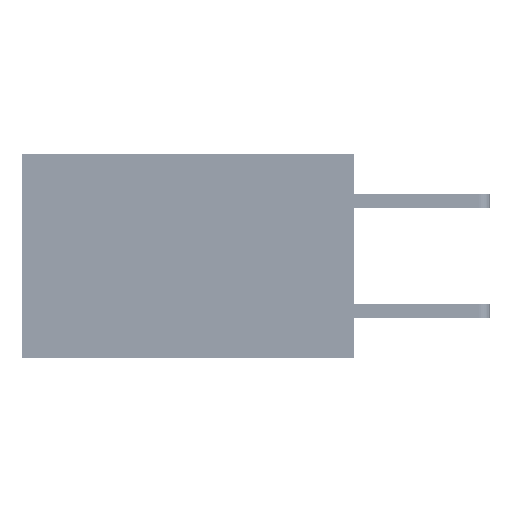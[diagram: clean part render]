
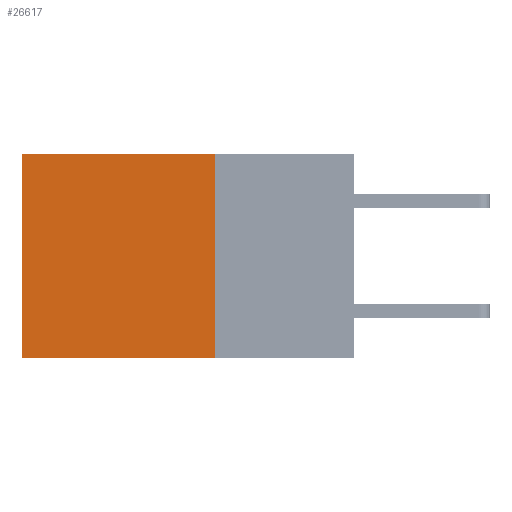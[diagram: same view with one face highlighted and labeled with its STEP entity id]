
A CAD part, left-side view. The second image highlights one B-rep face of the part: STEP entity #26617.
In plain terms, the highlighted planar face has unit normal (-1, 0, 0).
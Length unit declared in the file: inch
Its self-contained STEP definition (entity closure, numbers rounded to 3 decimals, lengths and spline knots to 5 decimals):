
#2583 = LINE ( 'NONE', #47488, #50290 ) ;
#2669 = CARTESIAN_POINT ( 'NONE',  ( 0.2875, 0.6, -0.37 ) ) ;
#3709 = EDGE_CURVE ( 'NONE', #24213, #41775, #29085, .T. ) ;
#3801 = CARTESIAN_POINT ( 'NONE',  ( 0.2875, 0.25, -0.37 ) ) ;
#5048 = DIRECTION ( 'NONE',  ( 0., 1., 0. ) ) ;
#6893 = ORIENTED_EDGE ( 'NONE', *, *, #13552, .F. ) ;
#9048 = LINE ( 'NONE', #33098, #9202 ) ;
#9202 = VECTOR ( 'NONE', #20428, 39.37008 ) ;
#13143 = ORIENTED_EDGE ( 'NONE', *, *, #35136, .T. ) ;
#13552 = EDGE_CURVE ( 'NONE', #24550, #24213, #2583, .T. ) ;
#14744 = VECTOR ( 'NONE', #5048, 39.37008 ) ;
#20428 = DIRECTION ( 'NONE',  ( 0., 0., -1. ) ) ;
#23697 = EDGE_CURVE ( 'NONE', #24550, #23934, #39280, .T. ) ;
#23934 = VERTEX_POINT ( 'NONE', #37385 ) ;
#24213 = VERTEX_POINT ( 'NONE', #3801 ) ;
#24550 = VERTEX_POINT ( 'NONE', #33618 ) ;
#26617 = ADVANCED_FACE ( 'NONE', ( #29527 ), #33771, .F. ) ;
#27905 = DIRECTION ( 'NONE',  ( 0., 1., 0. ) ) ;
#28575 = CARTESIAN_POINT ( 'NONE',  ( 0.2875, 0.25, -0.37 ) ) ;
#29085 = LINE ( 'NONE', #28575, #14744 ) ;
#29527 = FACE_OUTER_BOUND ( 'NONE', #48873, .T. ) ;
#33098 = CARTESIAN_POINT ( 'NONE',  ( 0.2875, 0.6, 0. ) ) ;
#33337 = AXIS2_PLACEMENT_3D ( 'NONE', #41442, #46450, #38251 ) ;
#33618 = CARTESIAN_POINT ( 'NONE',  ( 0.2875, 0.25, 0. ) ) ;
#33771 = PLANE ( 'NONE',  #33337 ) ;
#35136 = EDGE_CURVE ( 'NONE', #23934, #41775, #9048, .T. ) ;
#36944 = ORIENTED_EDGE ( 'NONE', *, *, #23697, .T. ) ;
#37385 = CARTESIAN_POINT ( 'NONE',  ( 0.2875, 0.6, 0. ) ) ;
#38251 = DIRECTION ( 'NONE',  ( 0., 0., -1. ) ) ;
#39280 = LINE ( 'NONE', #47197, #51724 ) ;
#41442 = CARTESIAN_POINT ( 'NONE',  ( 0.2875, 0.25, 0. ) ) ;
#41623 = ORIENTED_EDGE ( 'NONE', *, *, #3709, .F. ) ;
#41775 = VERTEX_POINT ( 'NONE', #2669 ) ;
#43006 = DIRECTION ( 'NONE',  ( 0., 0., -1. ) ) ;
#46450 = DIRECTION ( 'NONE',  ( 1., 0., 0. ) ) ;
#47197 = CARTESIAN_POINT ( 'NONE',  ( 0.2875, 0.25, 0. ) ) ;
#47488 = CARTESIAN_POINT ( 'NONE',  ( 0.2875, 0.25, 0. ) ) ;
#48873 = EDGE_LOOP ( 'NONE', ( #13143, #41623, #6893, #36944 ) ) ;
#50290 = VECTOR ( 'NONE', #43006, 39.37008 ) ;
#51724 = VECTOR ( 'NONE', #27905, 39.37008 ) ;
